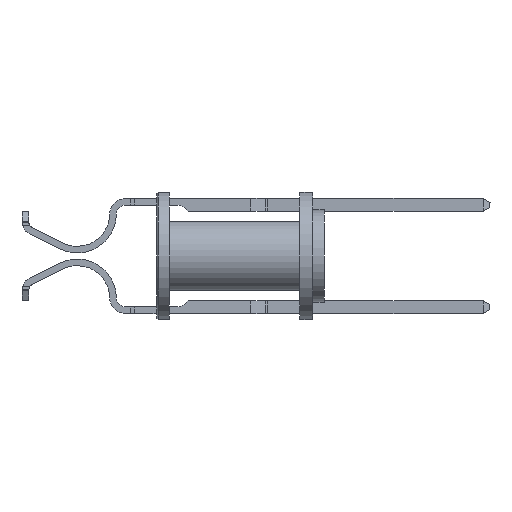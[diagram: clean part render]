
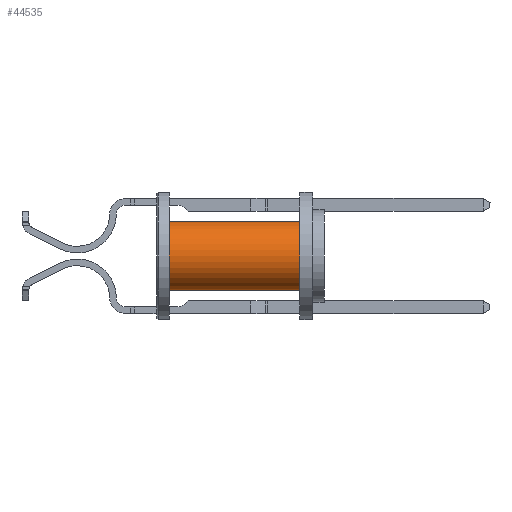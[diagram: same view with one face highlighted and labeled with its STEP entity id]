
A CAD part, left-side view. The second image highlights one B-rep face of the part: STEP entity #44535.
In plain terms, the highlighted cylindrical face has radius 1.727 mm (diameter 3.454 mm), a partial arc.
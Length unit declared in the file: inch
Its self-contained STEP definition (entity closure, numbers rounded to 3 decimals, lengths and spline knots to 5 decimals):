
#508 = EDGE_LOOP ( 'NONE', ( #19051, #23226, #15700, #7926 ) ) ;
#1857 = EDGE_CURVE ( 'NONE', #1885, #5708, #24579, .T. ) ;
#1885 = VERTEX_POINT ( 'NONE', #34138 ) ;
#1942 = CARTESIAN_POINT ( 'NONE',  ( 0., 0.28, 0.068 ) ) ;
#4645 = DIRECTION ( 'NONE',  ( 0., -1., 0. ) ) ;
#5708 = VERTEX_POINT ( 'NONE', #39357 ) ;
#7314 = VERTEX_POINT ( 'NONE', #22494 ) ;
#7926 = ORIENTED_EDGE ( 'NONE', *, *, #39484, .F. ) ;
#8184 = LINE ( 'NONE', #22835, #26307 ) ;
#9778 = LINE ( 'NONE', #16284, #27831 ) ;
#14787 = AXIS2_PLACEMENT_3D ( 'NONE', #38332, #17207, #41682 ) ;
#15523 = CYLINDRICAL_SURFACE ( 'NONE', #25196, 0.068 ) ;
#15686 = CARTESIAN_POINT ( 'NONE',  ( 0., 0.328, 0. ) ) ;
#15700 = ORIENTED_EDGE ( 'NONE', *, *, #1857, .T. ) ;
#16272 = CARTESIAN_POINT ( 'NONE',  ( 0., 0.025, 0. ) ) ;
#16284 = CARTESIAN_POINT ( 'NONE',  ( 0., 0.328, -0.068 ) ) ;
#17207 = DIRECTION ( 'NONE',  ( 0., 1., 0. ) ) ;
#17851 = FACE_OUTER_BOUND ( 'NONE', #508, .T. ) ;
#19051 = ORIENTED_EDGE ( 'NONE', *, *, #40182, .F. ) ;
#19935 = DIRECTION ( 'NONE',  ( 0., 0., 1. ) ) ;
#19939 = DIRECTION ( 'NONE',  ( 0., -1., 0. ) ) ;
#22440 = AXIS2_PLACEMENT_3D ( 'NONE', #16272, #40816, #19935 ) ;
#22494 = CARTESIAN_POINT ( 'NONE',  ( 0., 0.28, -0.068 ) ) ;
#22835 = CARTESIAN_POINT ( 'NONE',  ( 0., 0.328, 0.068 ) ) ;
#22995 = DIRECTION ( 'NONE',  ( 0., -1., 0. ) ) ;
#23226 = ORIENTED_EDGE ( 'NONE', *, *, #44524, .T. ) ;
#24579 = CIRCLE ( 'NONE', #22440, 0.068 ) ;
#25196 = AXIS2_PLACEMENT_3D ( 'NONE', #15686, #22995, #36960 ) ;
#26307 = VECTOR ( 'NONE', #4645, 39.37008 ) ;
#26442 = VERTEX_POINT ( 'NONE', #1942 ) ;
#27831 = VECTOR ( 'NONE', #19939, 39.37008 ) ;
#34138 = CARTESIAN_POINT ( 'NONE',  ( 0., 0.025, 0.068 ) ) ;
#34278 = CIRCLE ( 'NONE', #14787, 0.068 ) ;
#36960 = DIRECTION ( 'NONE',  ( 0., 0., -1. ) ) ;
#38332 = CARTESIAN_POINT ( 'NONE',  ( 0., 0.28, 0. ) ) ;
#39357 = CARTESIAN_POINT ( 'NONE',  ( 0., 0.025, -0.068 ) ) ;
#39484 = EDGE_CURVE ( 'NONE', #7314, #5708, #9778, .T. ) ;
#40182 = EDGE_CURVE ( 'NONE', #26442, #7314, #34278, .T. ) ;
#40816 = DIRECTION ( 'NONE',  ( 0., 1., 0. ) ) ;
#41682 = DIRECTION ( 'NONE',  ( 0., 0., 1. ) ) ;
#44524 = EDGE_CURVE ( 'NONE', #26442, #1885, #8184, .T. ) ;
#44535 = ADVANCED_FACE ( 'NONE', ( #17851 ), #15523, .T. ) ;
